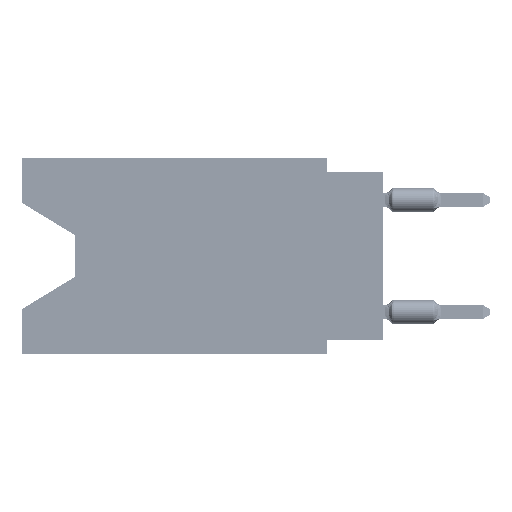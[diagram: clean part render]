
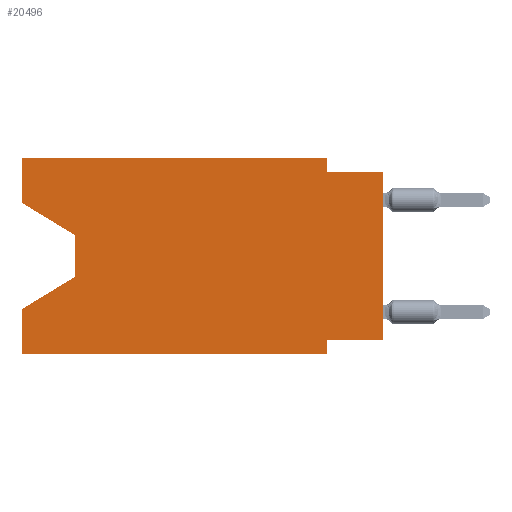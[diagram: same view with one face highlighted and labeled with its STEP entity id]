
A CAD part, left-side view. The second image highlights one B-rep face of the part: STEP entity #20496.
In plain terms, the highlighted planar face has unit normal (-1, 0, 0).
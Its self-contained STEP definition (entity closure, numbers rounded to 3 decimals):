
#1069 = VECTOR ( 'NONE', #82171, 1000. ) ;
#1955 = LINE ( 'NONE', #9619, #88564 ) ;
#2514 = ORIENTED_EDGE ( 'NONE', *, *, #103167, .T. ) ;
#3768 = EDGE_CURVE ( 'NONE', #79902, #91677, #4210, .T. ) ;
#4210 = LINE ( 'NONE', #70957, #53805 ) ;
#5704 = ORIENTED_EDGE ( 'NONE', *, *, #96958, .F. ) ;
#8601 = LINE ( 'NONE', #50717, #52530 ) ;
#8861 = DIRECTION ( 'NONE',  ( 0., -1., 0. ) ) ;
#9308 = EDGE_CURVE ( 'NONE', #96725, #87688, #17245, .T. ) ;
#9619 = CARTESIAN_POINT ( 'NONE',  ( 0., 0., 0. ) ) ;
#11028 = CARTESIAN_POINT ( 'NONE',  ( 0., 0., -8.255 ) ) ;
#11102 = LINE ( 'NONE', #52130, #11781 ) ;
#11313 = ORIENTED_EDGE ( 'NONE', *, *, #27110, .T. ) ;
#11781 = VECTOR ( 'NONE', #94292, 1000. ) ;
#11951 = CARTESIAN_POINT ( 'NONE',  ( 0., 16.383, -6.852 ) ) ;
#12657 = EDGE_CURVE ( 'NONE', #71695, #96725, #30433, .T. ) ;
#13990 = CARTESIAN_POINT ( 'NONE',  ( 0., 16.383, 0. ) ) ;
#14330 = CARTESIAN_POINT ( 'NONE',  ( 0., 0., -0.635 ) ) ;
#15451 = CARTESIAN_POINT ( 'NONE',  ( 0., 16.383, -8.89 ) ) ;
#17032 = EDGE_LOOP ( 'NONE', ( #50812, #100486, #107532, #35932, #2514, #89572, #5704, #11313, #23744, #17594, #56039, #18509 ) ) ;
#17245 = LINE ( 'NONE', #77960, #40624 ) ;
#17594 = ORIENTED_EDGE ( 'NONE', *, *, #25809, .F. ) ;
#18154 = CARTESIAN_POINT ( 'NONE',  ( 0., 2.54, 0. ) ) ;
#18509 = ORIENTED_EDGE ( 'NONE', *, *, #12657, .F. ) ;
#19241 = LINE ( 'NONE', #11028, #43998 ) ;
#20496 = ADVANCED_FACE ( 'NONE', ( #80331 ), #48566, .F. ) ;
#23744 = ORIENTED_EDGE ( 'NONE', *, *, #64706, .F. ) ;
#24165 = LINE ( 'NONE', #30769, #1069 ) ;
#24778 = LINE ( 'NONE', #58140, #102407 ) ;
#25809 = EDGE_CURVE ( 'NONE', #87688, #45726, #11102, .T. ) ;
#26749 = VECTOR ( 'NONE', #65399, 1000. ) ;
#27110 = EDGE_CURVE ( 'NONE', #66369, #96414, #1955, .T. ) ;
#27767 = CARTESIAN_POINT ( 'NONE',  ( 0., 2.54, -0.635 ) ) ;
#29887 = DIRECTION ( 'NONE',  ( 0., 0., 1. ) ) ;
#30433 = LINE ( 'NONE', #13990, #63639 ) ;
#30555 = DIRECTION ( 'NONE',  ( 1., 0., 0. ) ) ;
#30769 = CARTESIAN_POINT ( 'NONE',  ( 0., 13.97, -3.505 ) ) ;
#31130 = CARTESIAN_POINT ( 'NONE',  ( 0., 13.97, -3.505 ) ) ;
#31296 = VERTEX_POINT ( 'NONE', #31130 ) ;
#31627 = CARTESIAN_POINT ( 'NONE',  ( 0., 16.383, 0. ) ) ;
#33350 = AXIS2_PLACEMENT_3D ( 'NONE', #31627, #30555, #40364 ) ;
#35932 = ORIENTED_EDGE ( 'NONE', *, *, #87147, .F. ) ;
#36502 = DIRECTION ( 'NONE',  ( 0., 0.855, -0.519 ) ) ;
#37172 = EDGE_CURVE ( 'NONE', #71695, #31296, #24778, .T. ) ;
#37459 = CARTESIAN_POINT ( 'NONE',  ( 0., 0., -8.255 ) ) ;
#38578 = VERTEX_POINT ( 'NONE', #65750 ) ;
#40364 = DIRECTION ( 'NONE',  ( 0., 0., -1. ) ) ;
#40624 = VECTOR ( 'NONE', #84010, 1000. ) ;
#41172 = LINE ( 'NONE', #15451, #95535 ) ;
#42814 = CARTESIAN_POINT ( 'NONE',  ( 0., 16.383, -2.038 ) ) ;
#42997 = DIRECTION ( 'NONE',  ( 0., 0., 1. ) ) ;
#43998 = VECTOR ( 'NONE', #68495, 1000. ) ;
#44361 = VECTOR ( 'NONE', #89322, 1000. ) ;
#45726 = VERTEX_POINT ( 'NONE', #27767 ) ;
#48566 = PLANE ( 'NONE',  #33350 ) ;
#50717 = CARTESIAN_POINT ( 'NONE',  ( 0., 2.54, -8.89 ) ) ;
#50812 = ORIENTED_EDGE ( 'NONE', *, *, #37172, .T. ) ;
#52130 = CARTESIAN_POINT ( 'NONE',  ( 0., 2.54, 0. ) ) ;
#52530 = VECTOR ( 'NONE', #107669, 1000. ) ;
#53805 = VECTOR ( 'NONE', #36502, 1000. ) ;
#56039 = ORIENTED_EDGE ( 'NONE', *, *, #9308, .F. ) ;
#57542 = LINE ( 'NONE', #14330, #44361 ) ;
#58140 = CARTESIAN_POINT ( 'NONE',  ( 0., 16.383, -2.038 ) ) ;
#58790 = CARTESIAN_POINT ( 'NONE',  ( 0., 16.383, 0. ) ) ;
#63639 = VECTOR ( 'NONE', #29887, 1000. ) ;
#64706 = EDGE_CURVE ( 'NONE', #45726, #96414, #57542, .T. ) ;
#65399 = DIRECTION ( 'NONE',  ( 0., 0., 1. ) ) ;
#65750 = CARTESIAN_POINT ( 'NONE',  ( 0., 2.54, -8.255 ) ) ;
#66369 = VERTEX_POINT ( 'NONE', #37459 ) ;
#68321 = CARTESIAN_POINT ( 'NONE',  ( 0., 16.383, -8.89 ) ) ;
#68495 = DIRECTION ( 'NONE',  ( 0., 1., 0. ) ) ;
#70957 = CARTESIAN_POINT ( 'NONE',  ( 0., 13.97, -5.385 ) ) ;
#71695 = VERTEX_POINT ( 'NONE', #42814 ) ;
#72300 = VERTEX_POINT ( 'NONE', #89138 ) ;
#74680 = CARTESIAN_POINT ( 'NONE',  ( 0., 0., -0.635 ) ) ;
#77960 = CARTESIAN_POINT ( 'NONE',  ( 0., 16.383, 0. ) ) ;
#78350 = EDGE_CURVE ( 'NONE', #31296, #79902, #24165, .T. ) ;
#79902 = VERTEX_POINT ( 'NONE', #87041 ) ;
#80331 = FACE_OUTER_BOUND ( 'NONE', #17032, .T. ) ;
#82171 = DIRECTION ( 'NONE',  ( 0., 0., -1. ) ) ;
#83322 = DIRECTION ( 'NONE',  ( 0., -0.855, -0.519 ) ) ;
#84010 = DIRECTION ( 'NONE',  ( 0., -1., 0. ) ) ;
#84801 = EDGE_CURVE ( 'NONE', #38578, #72300, #8601, .T. ) ;
#87041 = CARTESIAN_POINT ( 'NONE',  ( 0., 13.97, -5.385 ) ) ;
#87147 = EDGE_CURVE ( 'NONE', #94478, #91677, #92181, .T. ) ;
#87688 = VERTEX_POINT ( 'NONE', #18154 ) ;
#88564 = VECTOR ( 'NONE', #42997, 1000. ) ;
#89138 = CARTESIAN_POINT ( 'NONE',  ( 0., 2.54, -8.89 ) ) ;
#89322 = DIRECTION ( 'NONE',  ( 0., -1., 0. ) ) ;
#89572 = ORIENTED_EDGE ( 'NONE', *, *, #84801, .F. ) ;
#91677 = VERTEX_POINT ( 'NONE', #11951 ) ;
#92181 = LINE ( 'NONE', #58790, #26749 ) ;
#94292 = DIRECTION ( 'NONE',  ( 0., 0., -1. ) ) ;
#94478 = VERTEX_POINT ( 'NONE', #68321 ) ;
#95535 = VECTOR ( 'NONE', #8861, 1000. ) ;
#96414 = VERTEX_POINT ( 'NONE', #74680 ) ;
#96725 = VERTEX_POINT ( 'NONE', #100816 ) ;
#96958 = EDGE_CURVE ( 'NONE', #66369, #38578, #19241, .T. ) ;
#100486 = ORIENTED_EDGE ( 'NONE', *, *, #78350, .T. ) ;
#100816 = CARTESIAN_POINT ( 'NONE',  ( 0., 16.383, 0. ) ) ;
#102407 = VECTOR ( 'NONE', #83322, 1000. ) ;
#103167 = EDGE_CURVE ( 'NONE', #94478, #72300, #41172, .T. ) ;
#107532 = ORIENTED_EDGE ( 'NONE', *, *, #3768, .T. ) ;
#107669 = DIRECTION ( 'NONE',  ( 0., 0., -1. ) ) ;
